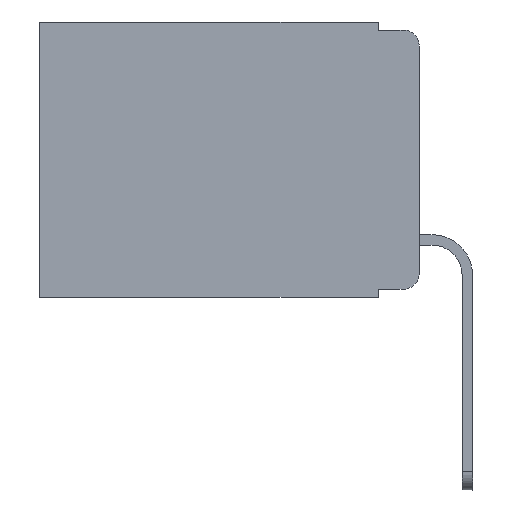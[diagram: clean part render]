
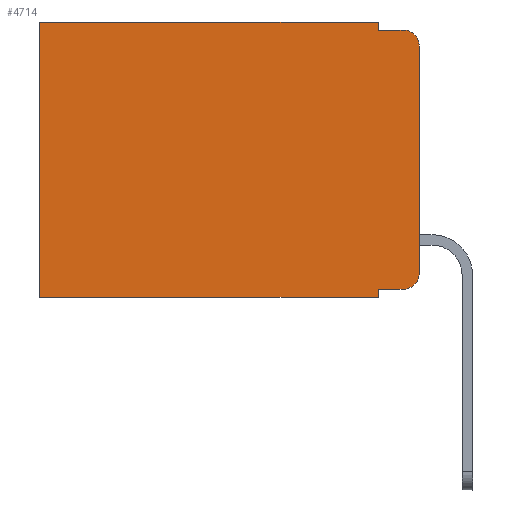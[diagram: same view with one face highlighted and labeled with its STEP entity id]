
A CAD part, left-side view. The second image highlights one B-rep face of the part: STEP entity #4714.
In plain terms, the highlighted planar face has unit normal (-1, 0, 0).
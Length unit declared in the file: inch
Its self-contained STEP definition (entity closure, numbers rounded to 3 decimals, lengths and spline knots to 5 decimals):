
#220 = VECTOR ( 'NONE', #4500, 39.37008 ) ;
#413 = CARTESIAN_POINT ( 'NONE',  ( 0.298, 0., -0.03 ) ) ;
#474 = VERTEX_POINT ( 'NONE', #7657 ) ;
#536 = VECTOR ( 'NONE', #2903, 39.37008 ) ;
#581 = DIRECTION ( 'NONE',  ( 0., 0., -1. ) ) ;
#624 = PLANE ( 'NONE',  #3787 ) ;
#651 = DIRECTION ( 'NONE',  ( 0., 0., -1. ) ) ;
#681 = ORIENTED_EDGE ( 'NONE', *, *, #6510, .F. ) ;
#760 = LINE ( 'NONE', #3690, #220 ) ;
#886 = VERTEX_POINT ( 'NONE', #6988 ) ;
#967 = DIRECTION ( 'NONE',  ( 0., 1., 0. ) ) ;
#1068 = LINE ( 'NONE', #4002, #6036 ) ;
#1169 = VERTEX_POINT ( 'NONE', #2367 ) ;
#1192 = EDGE_CURVE ( 'NONE', #3697, #3886, #1433, .T. ) ;
#1199 = DIRECTION ( 'NONE',  ( 0., 0., -1. ) ) ;
#1420 = CARTESIAN_POINT ( 'NONE',  ( 0.298, 0.051, 0. ) ) ;
#1433 = CIRCLE ( 'NONE', #7217, 0.02 ) ;
#1593 = DIRECTION ( 'NONE',  ( 0., 0., -1. ) ) ;
#1636 = EDGE_CURVE ( 'NONE', #1169, #2801, #1862, .T. ) ;
#1753 = CARTESIAN_POINT ( 'NONE',  ( 0.298, 0.473, 0. ) ) ;
#1755 = EDGE_CURVE ( 'NONE', #2335, #3886, #7660, .T. ) ;
#1837 = CARTESIAN_POINT ( 'NONE',  ( 0.298, 0.02, -0.03 ) ) ;
#1862 = LINE ( 'NONE', #8951, #6367 ) ;
#1928 = CARTESIAN_POINT ( 'NONE',  ( 0.298, 0., 0. ) ) ;
#2098 = LINE ( 'NONE', #1420, #9064 ) ;
#2155 = CARTESIAN_POINT ( 'NONE',  ( 0.298, 0., -0.313 ) ) ;
#2260 = ORIENTED_EDGE ( 'NONE', *, *, #5711, .T. ) ;
#2335 = VERTEX_POINT ( 'NONE', #8193 ) ;
#2367 = CARTESIAN_POINT ( 'NONE',  ( 0.298, 0.051, -0.333 ) ) ;
#2583 = ORIENTED_EDGE ( 'NONE', *, *, #7349, .F. ) ;
#2686 = CARTESIAN_POINT ( 'NONE',  ( 0.298, 0.02, -0.313 ) ) ;
#2801 = VERTEX_POINT ( 'NONE', #5312 ) ;
#2903 = DIRECTION ( 'NONE',  ( 0., 1., 0. ) ) ;
#2989 = CARTESIAN_POINT ( 'NONE',  ( 0.298, 0.473, 0. ) ) ;
#3064 = EDGE_CURVE ( 'NONE', #1169, #3082, #2098, .T. ) ;
#3082 = VERTEX_POINT ( 'NONE', #7814 ) ;
#3260 = ORIENTED_EDGE ( 'NONE', *, *, #1192, .T. ) ;
#3266 = LINE ( 'NONE', #6169, #4183 ) ;
#3338 = VECTOR ( 'NONE', #6414, 39.37008 ) ;
#3578 = CARTESIAN_POINT ( 'NONE',  ( 0.298, 0., -0.343 ) ) ;
#3690 = CARTESIAN_POINT ( 'NONE',  ( 0.298, 0., 0. ) ) ;
#3697 = VERTEX_POINT ( 'NONE', #413 ) ;
#3787 = AXIS2_PLACEMENT_3D ( 'NONE', #1928, #7742, #1199 ) ;
#3886 = VERTEX_POINT ( 'NONE', #5176 ) ;
#4002 = CARTESIAN_POINT ( 'NONE',  ( 0.298, 0.051, 0. ) ) ;
#4072 = ORIENTED_EDGE ( 'NONE', *, *, #7465, .T. ) ;
#4099 = DIRECTION ( 'NONE',  ( 0., 0., -1. ) ) ;
#4144 = ORIENTED_EDGE ( 'NONE', *, *, #3064, .F. ) ;
#4183 = VECTOR ( 'NONE', #967, 39.37008 ) ;
#4276 = EDGE_LOOP ( 'NONE', ( #681, #3260, #8151, #6154, #9331, #2260, #2583, #4144, #7863, #4072 ) ) ;
#4277 = FACE_OUTER_BOUND ( 'NONE', #4276, .T. ) ;
#4500 = DIRECTION ( 'NONE',  ( 0., 0., -1. ) ) ;
#4617 = LINE ( 'NONE', #2989, #4857 ) ;
#4714 = ADVANCED_FACE ( 'NONE', ( #4277 ), #624, .F. ) ;
#4857 = VECTOR ( 'NONE', #1593, 39.37008 ) ;
#5176 = CARTESIAN_POINT ( 'NONE',  ( 0.298, 0.02, -0.01 ) ) ;
#5283 = VERTEX_POINT ( 'NONE', #2155 ) ;
#5312 = CARTESIAN_POINT ( 'NONE',  ( 0.298, 0.02, -0.333 ) ) ;
#5345 = DIRECTION ( 'NONE',  ( 0., -1., 0. ) ) ;
#5452 = DIRECTION ( 'NONE',  ( 0., 0., -1. ) ) ;
#5711 = EDGE_CURVE ( 'NONE', #7148, #474, #4617, .T. ) ;
#6036 = VECTOR ( 'NONE', #4099, 39.37008 ) ;
#6154 = ORIENTED_EDGE ( 'NONE', *, *, #8147, .F. ) ;
#6169 = CARTESIAN_POINT ( 'NONE',  ( 0.298, 0., 0. ) ) ;
#6303 = DIRECTION ( 'NONE',  ( -1., 0., 0. ) ) ;
#6367 = VECTOR ( 'NONE', #5345, 39.37008 ) ;
#6414 = DIRECTION ( 'NONE',  ( 0., -1., 0. ) ) ;
#6510 = EDGE_CURVE ( 'NONE', #3697, #5283, #760, .T. ) ;
#6988 = CARTESIAN_POINT ( 'NONE',  ( 0.298, 0.051, 0. ) ) ;
#7148 = VERTEX_POINT ( 'NONE', #1753 ) ;
#7217 = AXIS2_PLACEMENT_3D ( 'NONE', #1837, #8273, #5452 ) ;
#7349 = EDGE_CURVE ( 'NONE', #3082, #474, #9367, .T. ) ;
#7465 = EDGE_CURVE ( 'NONE', #2801, #5283, #8019, .T. ) ;
#7657 = CARTESIAN_POINT ( 'NONE',  ( 0.298, 0.473, -0.343 ) ) ;
#7660 = LINE ( 'NONE', #8737, #3338 ) ;
#7742 = DIRECTION ( 'NONE',  ( 1., 0., 0. ) ) ;
#7814 = CARTESIAN_POINT ( 'NONE',  ( 0.298, 0.051, -0.343 ) ) ;
#7863 = ORIENTED_EDGE ( 'NONE', *, *, #1636, .T. ) ;
#8019 = CIRCLE ( 'NONE', #9201, 0.02 ) ;
#8147 = EDGE_CURVE ( 'NONE', #886, #2335, #1068, .T. ) ;
#8151 = ORIENTED_EDGE ( 'NONE', *, *, #1755, .F. ) ;
#8193 = CARTESIAN_POINT ( 'NONE',  ( 0.298, 0.051, -0.01 ) ) ;
#8273 = DIRECTION ( 'NONE',  ( -1., 0., 0. ) ) ;
#8588 = EDGE_CURVE ( 'NONE', #886, #7148, #3266, .T. ) ;
#8737 = CARTESIAN_POINT ( 'NONE',  ( 0.298, 0.051, -0.01 ) ) ;
#8951 = CARTESIAN_POINT ( 'NONE',  ( 0.298, 0.051, -0.333 ) ) ;
#9064 = VECTOR ( 'NONE', #651, 39.37008 ) ;
#9201 = AXIS2_PLACEMENT_3D ( 'NONE', #2686, #6303, #581 ) ;
#9331 = ORIENTED_EDGE ( 'NONE', *, *, #8588, .T. ) ;
#9367 = LINE ( 'NONE', #3578, #536 ) ;
